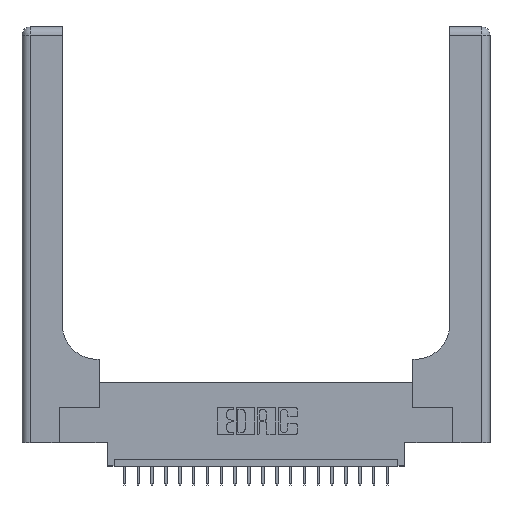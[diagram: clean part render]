
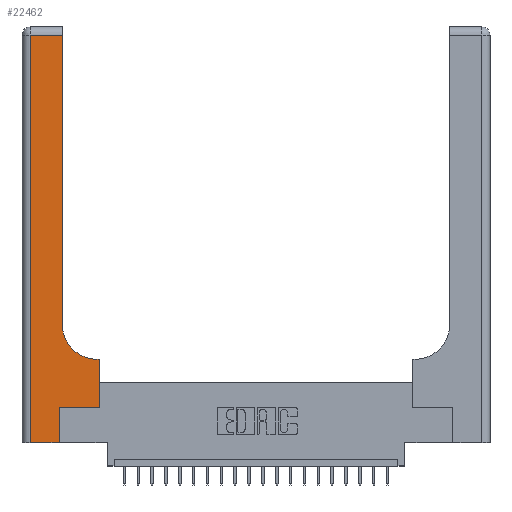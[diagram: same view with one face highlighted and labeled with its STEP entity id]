
A CAD part, top view. The second image highlights one B-rep face of the part: STEP entity #22462.
In plain terms, the highlighted planar face has unit normal (0, 0, 1).
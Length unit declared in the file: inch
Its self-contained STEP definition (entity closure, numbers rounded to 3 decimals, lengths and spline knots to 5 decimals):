
#2 = DIRECTION ( 'NONE',  ( 0., -1., 0. ) ) ;
#803 = LINE ( 'NONE', #15036, #21215 ) ;
#1276 = VERTEX_POINT ( 'NONE', #10946 ) ;
#1327 = LINE ( 'NONE', #1545, #9100 ) ;
#1370 = VERTEX_POINT ( 'NONE', #6297 ) ;
#1544 = EDGE_CURVE ( 'NONE', #11043, #1276, #15752, .T. ) ;
#1545 = CARTESIAN_POINT ( 'NONE',  ( 0., 0., 0.37 ) ) ;
#1677 = CIRCLE ( 'NONE', #15682, 0.25 ) ;
#2066 = CARTESIAN_POINT ( 'NONE',  ( 0.5415, 0.85, 0.37 ) ) ;
#2246 = VERTEX_POINT ( 'NONE', #13246 ) ;
#2897 = AXIS2_PLACEMENT_3D ( 'NONE', #5000, #5235, #19446 ) ;
#3533 = VERTEX_POINT ( 'NONE', #10140 ) ;
#3578 = ORIENTED_EDGE ( 'NONE', *, *, #1544, .T. ) ;
#3910 = LINE ( 'NONE', #12939, #13791 ) ;
#4193 = CARTESIAN_POINT ( 'NONE',  ( 0.2915, 0.85, 0.37 ) ) ;
#4390 = DIRECTION ( 'NONE',  ( -1., 0., 0. ) ) ;
#4764 = CARTESIAN_POINT ( 'NONE',  ( 0.06, 0., 0.37 ) ) ;
#4960 = CARTESIAN_POINT ( 'NONE',  ( 0.2915, 0.6, 0.37 ) ) ;
#5000 = CARTESIAN_POINT ( 'NONE',  ( 0., 3., 0.37 ) ) ;
#5086 = CARTESIAN_POINT ( 'NONE',  ( 0.2915, 3., 0.37 ) ) ;
#5222 = EDGE_CURVE ( 'NONE', #11187, #3533, #16175, .T. ) ;
#5235 = DIRECTION ( 'NONE',  ( 0., 0., -1. ) ) ;
#5348 = PLANE ( 'NONE',  #2897 ) ;
#5360 = CARTESIAN_POINT ( 'NONE',  ( 0.269, 0.25, 0.37 ) ) ;
#5448 = LINE ( 'NONE', #16737, #16859 ) ;
#6297 = CARTESIAN_POINT ( 'NONE',  ( 0.5585, 0.6, 0.37 ) ) ;
#6516 = VECTOR ( 'NONE', #15624, 39.37008 ) ;
#7951 = ORIENTED_EDGE ( 'NONE', *, *, #15013, .T. ) ;
#8422 = DIRECTION ( 'NONE',  ( 0., 1., 0. ) ) ;
#9100 = VECTOR ( 'NONE', #17685, 39.37008 ) ;
#9457 = DIRECTION ( 'NONE',  ( 1., 0., 0. ) ) ;
#10076 = ORIENTED_EDGE ( 'NONE', *, *, #20117, .T. ) ;
#10140 = CARTESIAN_POINT ( 'NONE',  ( 0.269, 0.25, 0.37 ) ) ;
#10946 = CARTESIAN_POINT ( 'NONE',  ( 0.2915, 2.94, 0.37 ) ) ;
#11043 = VERTEX_POINT ( 'NONE', #4193 ) ;
#11187 = VERTEX_POINT ( 'NONE', #20521 ) ;
#11342 = EDGE_CURVE ( 'NONE', #18073, #11187, #1327, .T. ) ;
#11871 = EDGE_CURVE ( 'NONE', #17122, #1370, #803, .T. ) ;
#12348 = ORIENTED_EDGE ( 'NONE', *, *, #5222, .T. ) ;
#12472 = VECTOR ( 'NONE', #15818, 39.37008 ) ;
#12939 = CARTESIAN_POINT ( 'NONE',  ( 0., 2.94, 0.37 ) ) ;
#13246 = CARTESIAN_POINT ( 'NONE',  ( 0.06, 2.94, 0.37 ) ) ;
#13791 = VECTOR ( 'NONE', #4390, 39.37008 ) ;
#13987 = CARTESIAN_POINT ( 'NONE',  ( 0.5415, 0.6, 0.37 ) ) ;
#14203 = EDGE_LOOP ( 'NONE', ( #3578, #19018, #10076, #22503, #12348, #21567, #18221, #7951, #21665 ) ) ;
#15013 = EDGE_CURVE ( 'NONE', #1370, #19160, #22649, .T. ) ;
#15036 = CARTESIAN_POINT ( 'NONE',  ( 0.5585, 0.25, 0.37 ) ) ;
#15624 = DIRECTION ( 'NONE',  ( -1., 0., 0. ) ) ;
#15682 = AXIS2_PLACEMENT_3D ( 'NONE', #2066, #16677, #9457 ) ;
#15752 = LINE ( 'NONE', #5086, #19237 ) ;
#15818 = DIRECTION ( 'NONE',  ( 0., 1., 0. ) ) ;
#16175 = LINE ( 'NONE', #23036, #12472 ) ;
#16677 = DIRECTION ( 'NONE',  ( 0., 0., -1. ) ) ;
#16737 = CARTESIAN_POINT ( 'NONE',  ( 0.06, 3., 0.37 ) ) ;
#16859 = VECTOR ( 'NONE', #2, 39.37008 ) ;
#17122 = VERTEX_POINT ( 'NONE', #22557 ) ;
#17353 = EDGE_CURVE ( 'NONE', #1276, #2246, #3910, .T. ) ;
#17685 = DIRECTION ( 'NONE',  ( 1., 0., 0. ) ) ;
#17910 = EDGE_CURVE ( 'NONE', #3533, #17122, #21599, .T. ) ;
#18073 = VERTEX_POINT ( 'NONE', #4764 ) ;
#18221 = ORIENTED_EDGE ( 'NONE', *, *, #11871, .T. ) ;
#18939 = DIRECTION ( 'NONE',  ( 0., 1., 0. ) ) ;
#19018 = ORIENTED_EDGE ( 'NONE', *, *, #17353, .T. ) ;
#19108 = VECTOR ( 'NONE', #21479, 39.37008 ) ;
#19160 = VERTEX_POINT ( 'NONE', #13987 ) ;
#19237 = VECTOR ( 'NONE', #8422, 39.37008 ) ;
#19446 = DIRECTION ( 'NONE',  ( -1., 0., 0. ) ) ;
#19647 = EDGE_CURVE ( 'NONE', #19160, #11043, #1677, .T. ) ;
#20117 = EDGE_CURVE ( 'NONE', #2246, #18073, #5448, .T. ) ;
#20521 = CARTESIAN_POINT ( 'NONE',  ( 0.269, 0., 0.37 ) ) ;
#21215 = VECTOR ( 'NONE', #18939, 39.37008 ) ;
#21238 = FACE_OUTER_BOUND ( 'NONE', #14203, .T. ) ;
#21479 = DIRECTION ( 'NONE',  ( 1., 0., 0. ) ) ;
#21567 = ORIENTED_EDGE ( 'NONE', *, *, #17910, .T. ) ;
#21599 = LINE ( 'NONE', #5360, #19108 ) ;
#21665 = ORIENTED_EDGE ( 'NONE', *, *, #19647, .T. ) ;
#22462 = ADVANCED_FACE ( 'NONE', ( #21238 ), #5348, .F. ) ;
#22503 = ORIENTED_EDGE ( 'NONE', *, *, #11342, .T. ) ;
#22557 = CARTESIAN_POINT ( 'NONE',  ( 0.5585, 0.25, 0.37 ) ) ;
#22649 = LINE ( 'NONE', #4960, #6516 ) ;
#23036 = CARTESIAN_POINT ( 'NONE',  ( 0.269, 0., 0.37 ) ) ;
